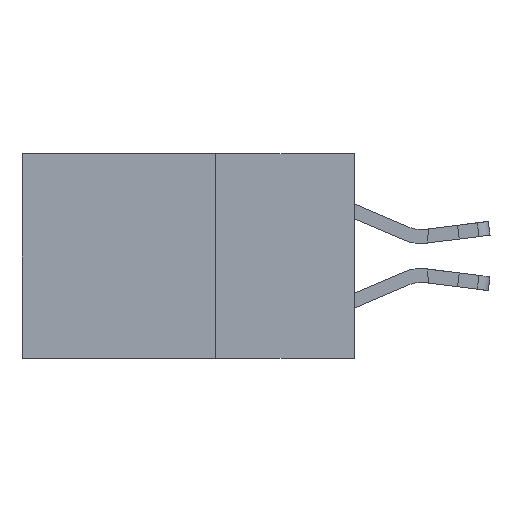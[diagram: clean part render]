
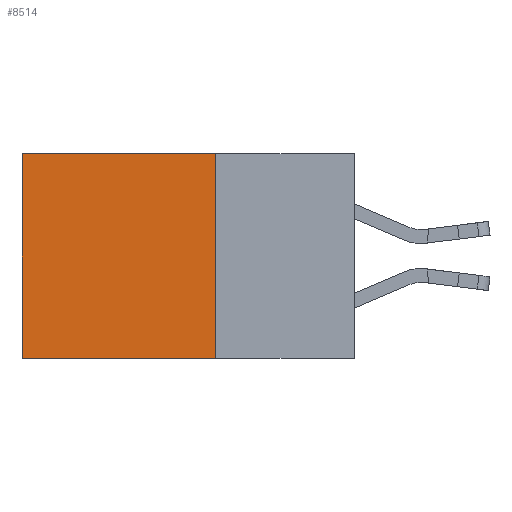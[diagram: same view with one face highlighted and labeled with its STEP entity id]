
A CAD part, left-side view. The second image highlights one B-rep face of the part: STEP entity #8514.
In plain terms, the highlighted planar face has unit normal (-1, 0, 0).
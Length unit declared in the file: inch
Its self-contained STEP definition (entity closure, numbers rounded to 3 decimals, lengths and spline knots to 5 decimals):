
#2015 = EDGE_CURVE ( 'NONE', #8195, #4683, #11368, .T. ) ;
#2404 = CARTESIAN_POINT ( 'NONE',  ( 0.2615, 0.25, -0.37 ) ) ;
#2584 = VECTOR ( 'NONE', #3447, 39.37008 ) ;
#2592 = EDGE_CURVE ( 'NONE', #12260, #4683, #8556, .T. ) ;
#2736 = DIRECTION ( 'NONE',  ( 0., 0., -1. ) ) ;
#2811 = FACE_OUTER_BOUND ( 'NONE', #11333, .T. ) ;
#3447 = DIRECTION ( 'NONE',  ( 0., 0., -1. ) ) ;
#3613 = ORIENTED_EDGE ( 'NONE', *, *, #9711, .T. ) ;
#3654 = DIRECTION ( 'NONE',  ( 0., 0., -1. ) ) ;
#3908 = CARTESIAN_POINT ( 'NONE',  ( 0.2615, 0.25, -0.37 ) ) ;
#4241 = DIRECTION ( 'NONE',  ( 0., 1., 0. ) ) ;
#4658 = CARTESIAN_POINT ( 'NONE',  ( 0.2615, 0.25, -0.37 ) ) ;
#4683 = VERTEX_POINT ( 'NONE', #6075 ) ;
#4698 = ORIENTED_EDGE ( 'NONE', *, *, #5890, .F. ) ;
#4811 = VECTOR ( 'NONE', #4241, 39.37008 ) ;
#4933 = DIRECTION ( 'NONE',  ( 0., 1., 0. ) ) ;
#5235 = VECTOR ( 'NONE', #3654, 39.37008 ) ;
#5890 = EDGE_CURVE ( 'NONE', #11930, #8195, #12945, .T. ) ;
#6075 = CARTESIAN_POINT ( 'NONE',  ( 0.2615, 0.6, -0.37 ) ) ;
#6655 = ORIENTED_EDGE ( 'NONE', *, *, #2592, .T. ) ;
#6906 = CARTESIAN_POINT ( 'NONE',  ( 0.2615, 0.25, 0. ) ) ;
#7654 = AXIS2_PLACEMENT_3D ( 'NONE', #4658, #8909, #2736 ) ;
#7691 = CARTESIAN_POINT ( 'NONE',  ( 0.2615, 0.6, -0.37 ) ) ;
#8195 = VERTEX_POINT ( 'NONE', #9841 ) ;
#8514 = ADVANCED_FACE ( 'NONE', ( #2811 ), #12968, .F. ) ;
#8556 = LINE ( 'NONE', #7691, #2584 ) ;
#8909 = DIRECTION ( 'NONE',  ( 1., 0., 0. ) ) ;
#9711 = EDGE_CURVE ( 'NONE', #11930, #12260, #13114, .T. ) ;
#9841 = CARTESIAN_POINT ( 'NONE',  ( 0.2615, 0.25, -0.37 ) ) ;
#9901 = CARTESIAN_POINT ( 'NONE',  ( 0.2615, 0.25, 0. ) ) ;
#10487 = CARTESIAN_POINT ( 'NONE',  ( 0.2615, 0.6, 0. ) ) ;
#11065 = VECTOR ( 'NONE', #4933, 39.37008 ) ;
#11333 = EDGE_LOOP ( 'NONE', ( #6655, #11575, #4698, #3613 ) ) ;
#11368 = LINE ( 'NONE', #2404, #4811 ) ;
#11575 = ORIENTED_EDGE ( 'NONE', *, *, #2015, .F. ) ;
#11930 = VERTEX_POINT ( 'NONE', #6906 ) ;
#12260 = VERTEX_POINT ( 'NONE', #10487 ) ;
#12945 = LINE ( 'NONE', #3908, #5235 ) ;
#12968 = PLANE ( 'NONE',  #7654 ) ;
#13114 = LINE ( 'NONE', #9901, #11065 ) ;
